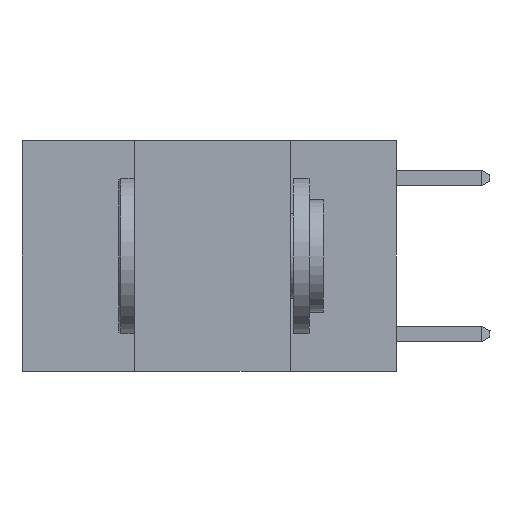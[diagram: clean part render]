
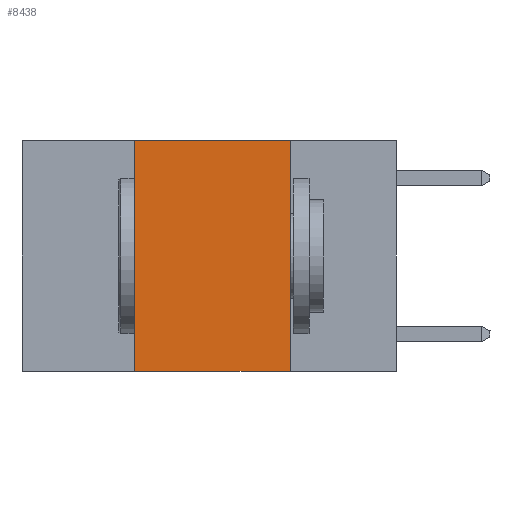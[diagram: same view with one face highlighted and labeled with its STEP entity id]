
A CAD part, left-side view. The second image highlights one B-rep face of the part: STEP entity #8438.
In plain terms, the highlighted planar face has unit normal (-1, 0, 0).
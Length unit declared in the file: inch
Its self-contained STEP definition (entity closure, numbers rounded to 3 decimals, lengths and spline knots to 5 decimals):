
#474 = DIRECTION ( 'NONE',  ( 0., 0., -1. ) ) ;
#617 = FACE_OUTER_BOUND ( 'NONE', #1360, .T. ) ;
#1212 = VECTOR ( 'NONE', #3222, 39.37008 ) ;
#1347 = VERTEX_POINT ( 'NONE', #11760 ) ;
#1360 = EDGE_LOOP ( 'NONE', ( #13154, #7905, #13724, #13850 ) ) ;
#1457 = CARTESIAN_POINT ( 'NONE',  ( 0., 0.17, 0. ) ) ;
#1489 = VECTOR ( 'NONE', #12336, 39.37008 ) ;
#1911 = VERTEX_POINT ( 'NONE', #2037 ) ;
#1943 = CARTESIAN_POINT ( 'NONE',  ( 0., 0.6, -0.37 ) ) ;
#2037 = CARTESIAN_POINT ( 'NONE',  ( 0., 0.17, -0.37 ) ) ;
#2279 = VERTEX_POINT ( 'NONE', #11280 ) ;
#2304 = CARTESIAN_POINT ( 'NONE',  ( 0., 0.6, 0. ) ) ;
#2787 = LINE ( 'NONE', #2304, #9102 ) ;
#3222 = DIRECTION ( 'NONE',  ( 0., -1., 0. ) ) ;
#3288 = EDGE_CURVE ( 'NONE', #1347, #1911, #7801, .T. ) ;
#6694 = CARTESIAN_POINT ( 'NONE',  ( 0., 0.6, 0. ) ) ;
#6898 = EDGE_CURVE ( 'NONE', #13658, #1911, #8436, .T. ) ;
#7801 = LINE ( 'NONE', #1943, #1212 ) ;
#7895 = DIRECTION ( 'NONE',  ( 1., 0., 0. ) ) ;
#7905 = ORIENTED_EDGE ( 'NONE', *, *, #8860, .F. ) ;
#8436 = LINE ( 'NONE', #14112, #11298 ) ;
#8438 = ADVANCED_FACE ( 'NONE', ( #617 ), #13913, .F. ) ;
#8860 = EDGE_CURVE ( 'NONE', #2279, #13658, #2787, .T. ) ;
#9102 = VECTOR ( 'NONE', #13257, 39.37008 ) ;
#10914 = LINE ( 'NONE', #11118, #1489 ) ;
#11118 = CARTESIAN_POINT ( 'NONE',  ( 0., 0.42, 0. ) ) ;
#11280 = CARTESIAN_POINT ( 'NONE',  ( 0., 0.42, 0. ) ) ;
#11298 = VECTOR ( 'NONE', #15299, 39.37008 ) ;
#11760 = CARTESIAN_POINT ( 'NONE',  ( 0., 0.42, -0.37 ) ) ;
#11957 = AXIS2_PLACEMENT_3D ( 'NONE', #6694, #7895, #474 ) ;
#12336 = DIRECTION ( 'NONE',  ( 0., 0., 1. ) ) ;
#12365 = EDGE_CURVE ( 'NONE', #1347, #2279, #10914, .T. ) ;
#13154 = ORIENTED_EDGE ( 'NONE', *, *, #6898, .F. ) ;
#13257 = DIRECTION ( 'NONE',  ( 0., -1., 0. ) ) ;
#13658 = VERTEX_POINT ( 'NONE', #1457 ) ;
#13724 = ORIENTED_EDGE ( 'NONE', *, *, #12365, .F. ) ;
#13850 = ORIENTED_EDGE ( 'NONE', *, *, #3288, .T. ) ;
#13913 = PLANE ( 'NONE',  #11957 ) ;
#14112 = CARTESIAN_POINT ( 'NONE',  ( 0., 0.17, 0. ) ) ;
#15299 = DIRECTION ( 'NONE',  ( 0., 0., -1. ) ) ;
